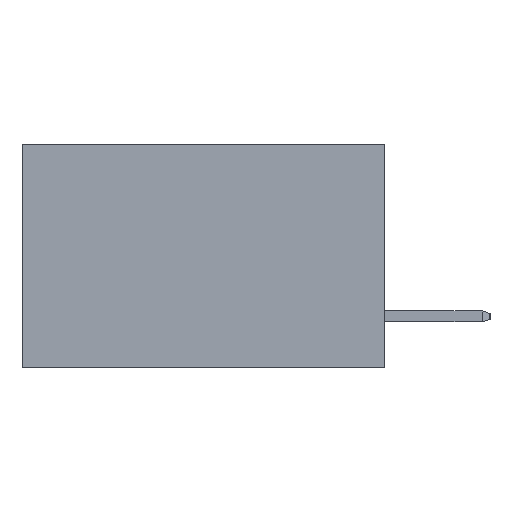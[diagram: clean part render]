
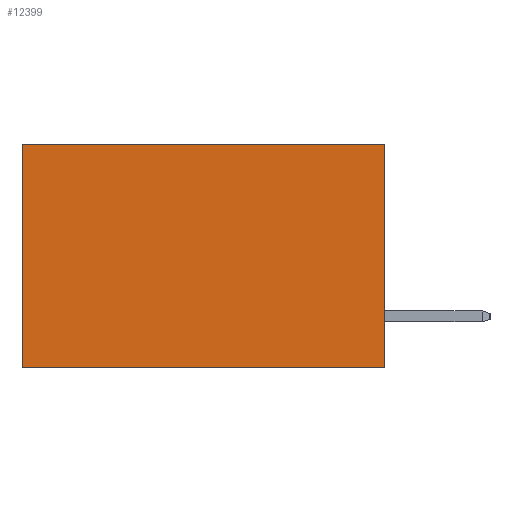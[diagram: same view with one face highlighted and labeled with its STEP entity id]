
A CAD part, left-side view. The second image highlights one B-rep face of the part: STEP entity #12399.
In plain terms, the highlighted planar face has unit normal (-1, 0, 0).
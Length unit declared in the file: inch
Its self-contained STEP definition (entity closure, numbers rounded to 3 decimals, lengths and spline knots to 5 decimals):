
#764 = CARTESIAN_POINT ( 'NONE',  ( 0.2615, 0.6, -0.37 ) ) ;
#1696 = VERTEX_POINT ( 'NONE', #15561 ) ;
#1853 = CARTESIAN_POINT ( 'NONE',  ( 0.2615, 0.6, 0. ) ) ;
#2235 = EDGE_LOOP ( 'NONE', ( #5114, #14938, #2823, #6349 ) ) ;
#2789 = VERTEX_POINT ( 'NONE', #4700 ) ;
#2823 = ORIENTED_EDGE ( 'NONE', *, *, #5484, .F. ) ;
#3274 = EDGE_CURVE ( 'NONE', #10855, #1696, #9869, .T. ) ;
#3373 = EDGE_CURVE ( 'NONE', #2789, #1696, #5340, .T. ) ;
#3718 = DIRECTION ( 'NONE',  ( 1., 0., 0. ) ) ;
#4700 = CARTESIAN_POINT ( 'NONE',  ( 0.2615, 0., -0.37 ) ) ;
#4790 = CARTESIAN_POINT ( 'NONE',  ( 0.2615, 0., 0. ) ) ;
#5105 = VERTEX_POINT ( 'NONE', #4790 ) ;
#5114 = ORIENTED_EDGE ( 'NONE', *, *, #3274, .T. ) ;
#5340 = LINE ( 'NONE', #6494, #8344 ) ;
#5484 = EDGE_CURVE ( 'NONE', #5105, #2789, #15655, .T. ) ;
#6261 = FACE_OUTER_BOUND ( 'NONE', #2235, .T. ) ;
#6334 = DIRECTION ( 'NONE',  ( 0., 0., -1. ) ) ;
#6336 = CARTESIAN_POINT ( 'NONE',  ( 0.2615, 0., -0.37 ) ) ;
#6349 = ORIENTED_EDGE ( 'NONE', *, *, #6445, .T. ) ;
#6445 = EDGE_CURVE ( 'NONE', #5105, #10855, #11674, .T. ) ;
#6494 = CARTESIAN_POINT ( 'NONE',  ( 0.2615, 0., -0.37 ) ) ;
#8344 = VECTOR ( 'NONE', #14543, 39.37008 ) ;
#8448 = VECTOR ( 'NONE', #11119, 39.37008 ) ;
#9263 = VECTOR ( 'NONE', #14204, 39.37008 ) ;
#9869 = LINE ( 'NONE', #764, #15878 ) ;
#10855 = VERTEX_POINT ( 'NONE', #1853 ) ;
#11119 = DIRECTION ( 'NONE',  ( 0., 1., 0. ) ) ;
#11306 = PLANE ( 'NONE',  #13557 ) ;
#11674 = LINE ( 'NONE', #12361, #8448 ) ;
#12361 = CARTESIAN_POINT ( 'NONE',  ( 0.2615, 0., 0. ) ) ;
#12399 = ADVANCED_FACE ( 'NONE', ( #6261 ), #11306, .F. ) ;
#12509 = DIRECTION ( 'NONE',  ( 0., 0., -1. ) ) ;
#12988 = CARTESIAN_POINT ( 'NONE',  ( 0.2615, 0., -0.37 ) ) ;
#13557 = AXIS2_PLACEMENT_3D ( 'NONE', #6336, #3718, #12509 ) ;
#14204 = DIRECTION ( 'NONE',  ( 0., 0., -1. ) ) ;
#14543 = DIRECTION ( 'NONE',  ( 0., 1., 0. ) ) ;
#14938 = ORIENTED_EDGE ( 'NONE', *, *, #3373, .F. ) ;
#15561 = CARTESIAN_POINT ( 'NONE',  ( 0.2615, 0.6, -0.37 ) ) ;
#15655 = LINE ( 'NONE', #12988, #9263 ) ;
#15878 = VECTOR ( 'NONE', #6334, 39.37008 ) ;
